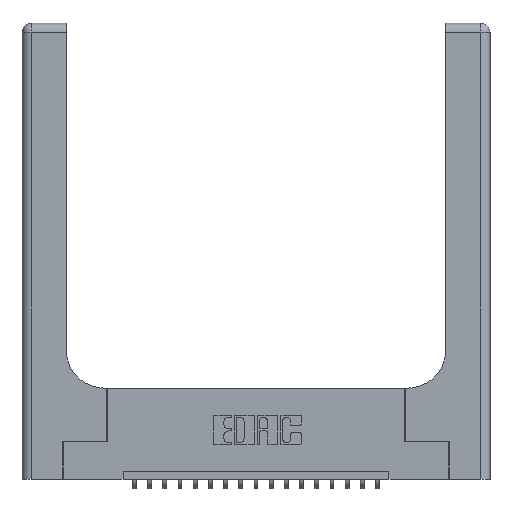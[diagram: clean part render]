
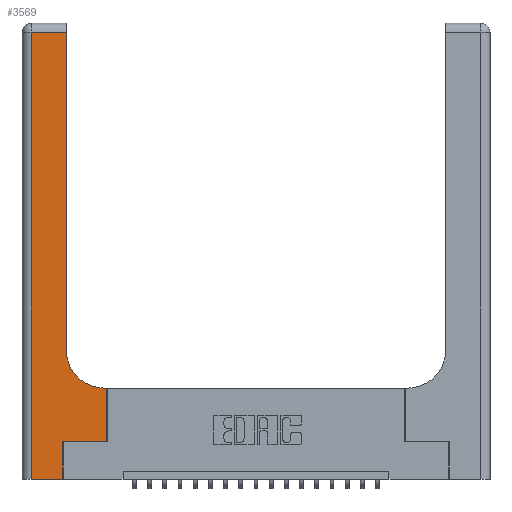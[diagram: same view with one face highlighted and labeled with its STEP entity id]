
A CAD part, top view. The second image highlights one B-rep face of the part: STEP entity #3569.
In plain terms, the highlighted planar face has unit normal (0, 0, 1).
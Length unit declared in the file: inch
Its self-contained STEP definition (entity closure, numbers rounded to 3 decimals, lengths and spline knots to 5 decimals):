
#1154 = ORIENTED_EDGE ( 'NONE', *, *, #11202, .T. ) ;
#1178 = DIRECTION ( 'NONE',  ( 0., 1., 0. ) ) ;
#1601 = EDGE_CURVE ( 'NONE', #2591, #14980, #5527, .T. ) ;
#1655 = EDGE_LOOP ( 'NONE', ( #1810, #5945, #1154, #3801, #18914, #16326, #3219, #3293, #11927 ) ) ;
#1810 = ORIENTED_EDGE ( 'NONE', *, *, #1601, .T. ) ;
#1834 = CARTESIAN_POINT ( 'NONE',  ( 0., 0., 0.37 ) ) ;
#2008 = DIRECTION ( 'NONE',  ( -1., 0., 0. ) ) ;
#2463 = EDGE_CURVE ( 'NONE', #14171, #9720, #5772, .T. ) ;
#2591 = VERTEX_POINT ( 'NONE', #11983 ) ;
#2892 = CARTESIAN_POINT ( 'NONE',  ( 0.269, 0., 0.37 ) ) ;
#2944 = CIRCLE ( 'NONE', #20236, 0.25 ) ;
#2976 = EDGE_CURVE ( 'NONE', #14980, #3665, #17093, .T. ) ;
#3219 = ORIENTED_EDGE ( 'NONE', *, *, #11943, .T. ) ;
#3293 = ORIENTED_EDGE ( 'NONE', *, *, #4633, .T. ) ;
#3569 = ADVANCED_FACE ( 'NONE', ( #17324 ), #14013, .F. ) ;
#3665 = VERTEX_POINT ( 'NONE', #19668 ) ;
#3801 = ORIENTED_EDGE ( 'NONE', *, *, #2463, .T. ) ;
#3866 = CARTESIAN_POINT ( 'NONE',  ( 0.2915, 2.94, 0.37 ) ) ;
#4091 = AXIS2_PLACEMENT_3D ( 'NONE', #7241, #8951, #15543 ) ;
#4601 = VERTEX_POINT ( 'NONE', #20885 ) ;
#4615 = VERTEX_POINT ( 'NONE', #20812 ) ;
#4633 = EDGE_CURVE ( 'NONE', #11044, #4615, #5126, .T. ) ;
#4772 = DIRECTION ( 'NONE',  ( 1., 0., 0. ) ) ;
#5126 = LINE ( 'NONE', #14177, #19589 ) ;
#5207 = CARTESIAN_POINT ( 'NONE',  ( 0.5415, 0.85, 0.37 ) ) ;
#5527 = LINE ( 'NONE', #6118, #11492 ) ;
#5772 = LINE ( 'NONE', #1834, #18423 ) ;
#5945 = ORIENTED_EDGE ( 'NONE', *, *, #2976, .T. ) ;
#6118 = CARTESIAN_POINT ( 'NONE',  ( 0.2915, 3., 0.37 ) ) ;
#6171 = CARTESIAN_POINT ( 'NONE',  ( 0.269, 0.25, 0.37 ) ) ;
#7028 = DIRECTION ( 'NONE',  ( 1., 0., 0. ) ) ;
#7241 = CARTESIAN_POINT ( 'NONE',  ( 0., 3., 0.37 ) ) ;
#7733 = CARTESIAN_POINT ( 'NONE',  ( 0.5585, 0.6, 0.37 ) ) ;
#8306 = DIRECTION ( 'NONE',  ( 0., 1., 0. ) ) ;
#8951 = DIRECTION ( 'NONE',  ( 0., 0., -1. ) ) ;
#9720 = VERTEX_POINT ( 'NONE', #2892 ) ;
#9986 = CARTESIAN_POINT ( 'NONE',  ( 0.06, 0., 0.37 ) ) ;
#9990 = EDGE_CURVE ( 'NONE', #9720, #19657, #19503, .T. ) ;
#10251 = CARTESIAN_POINT ( 'NONE',  ( 0., 2.94, 0.37 ) ) ;
#10924 = LINE ( 'NONE', #17986, #17369 ) ;
#11044 = VERTEX_POINT ( 'NONE', #7733 ) ;
#11202 = EDGE_CURVE ( 'NONE', #3665, #14171, #15336, .T. ) ;
#11492 = VECTOR ( 'NONE', #1178, 39.37008 ) ;
#11752 = VECTOR ( 'NONE', #4772, 39.37008 ) ;
#11872 = DIRECTION ( 'NONE',  ( 1., 0., 0. ) ) ;
#11927 = ORIENTED_EDGE ( 'NONE', *, *, #17840, .T. ) ;
#11943 = EDGE_CURVE ( 'NONE', #4601, #11044, #10924, .T. ) ;
#11983 = CARTESIAN_POINT ( 'NONE',  ( 0.2915, 0.85, 0.37 ) ) ;
#12242 = VECTOR ( 'NONE', #21242, 39.37008 ) ;
#14013 = PLANE ( 'NONE',  #4091 ) ;
#14171 = VERTEX_POINT ( 'NONE', #9986 ) ;
#14177 = CARTESIAN_POINT ( 'NONE',  ( 0.2915, 0.6, 0.37 ) ) ;
#14980 = VERTEX_POINT ( 'NONE', #3866 ) ;
#15094 = DIRECTION ( 'NONE',  ( 0., 1., 0. ) ) ;
#15336 = LINE ( 'NONE', #19645, #12242 ) ;
#15365 = CARTESIAN_POINT ( 'NONE',  ( 0.269, 0.25, 0.37 ) ) ;
#15543 = DIRECTION ( 'NONE',  ( -1., 0., 0. ) ) ;
#16326 = ORIENTED_EDGE ( 'NONE', *, *, #18088, .T. ) ;
#16650 = LINE ( 'NONE', #6171, #11752 ) ;
#16770 = DIRECTION ( 'NONE',  ( 0., 0., -1. ) ) ;
#17093 = LINE ( 'NONE', #10251, #17618 ) ;
#17324 = FACE_OUTER_BOUND ( 'NONE', #1655, .T. ) ;
#17369 = VECTOR ( 'NONE', #8306, 39.37008 ) ;
#17618 = VECTOR ( 'NONE', #2008, 39.37008 ) ;
#17840 = EDGE_CURVE ( 'NONE', #4615, #2591, #2944, .T. ) ;
#17986 = CARTESIAN_POINT ( 'NONE',  ( 0.5585, 0.25, 0.37 ) ) ;
#18088 = EDGE_CURVE ( 'NONE', #19657, #4601, #16650, .T. ) ;
#18423 = VECTOR ( 'NONE', #7028, 39.37008 ) ;
#18914 = ORIENTED_EDGE ( 'NONE', *, *, #9990, .T. ) ;
#19269 = VECTOR ( 'NONE', #15094, 39.37008 ) ;
#19503 = LINE ( 'NONE', #21447, #19269 ) ;
#19589 = VECTOR ( 'NONE', #20746, 39.37008 ) ;
#19645 = CARTESIAN_POINT ( 'NONE',  ( 0.06, 3., 0.37 ) ) ;
#19657 = VERTEX_POINT ( 'NONE', #15365 ) ;
#19668 = CARTESIAN_POINT ( 'NONE',  ( 0.06, 2.94, 0.37 ) ) ;
#20236 = AXIS2_PLACEMENT_3D ( 'NONE', #5207, #16770, #11872 ) ;
#20746 = DIRECTION ( 'NONE',  ( -1., 0., 0. ) ) ;
#20812 = CARTESIAN_POINT ( 'NONE',  ( 0.5415, 0.6, 0.37 ) ) ;
#20885 = CARTESIAN_POINT ( 'NONE',  ( 0.5585, 0.25, 0.37 ) ) ;
#21242 = DIRECTION ( 'NONE',  ( 0., -1., 0. ) ) ;
#21447 = CARTESIAN_POINT ( 'NONE',  ( 0.269, 0., 0.37 ) ) ;
